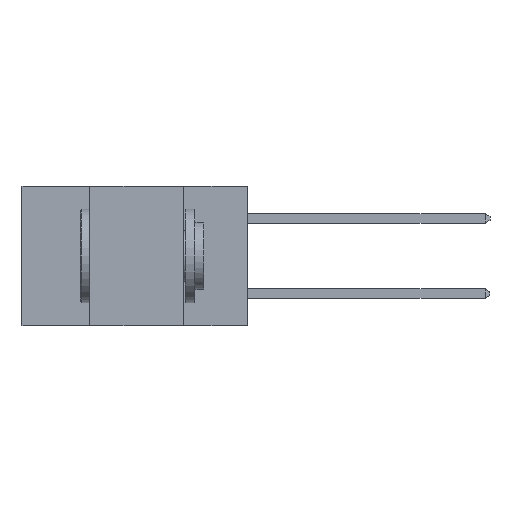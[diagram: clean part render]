
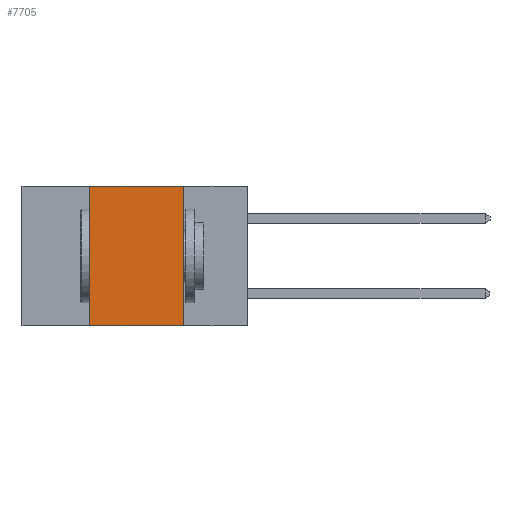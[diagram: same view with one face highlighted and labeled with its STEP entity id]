
A CAD part, left-side view. The second image highlights one B-rep face of the part: STEP entity #7705.
In plain terms, the highlighted planar face has unit normal (-1, 0, 0).
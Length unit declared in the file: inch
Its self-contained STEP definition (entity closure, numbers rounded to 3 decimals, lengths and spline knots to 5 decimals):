
#313 = CARTESIAN_POINT ( 'NONE',  ( 0., 0.42, 0. ) ) ;
#503 = LINE ( 'NONE', #12919, #856 ) ;
#856 = VECTOR ( 'NONE', #7271, 39.37008 ) ;
#1148 = CARTESIAN_POINT ( 'NONE',  ( 0., 0.6, 0. ) ) ;
#1267 = DIRECTION ( 'NONE',  ( 0., -1., 0. ) ) ;
#2216 = ORIENTED_EDGE ( 'NONE', *, *, #10490, .T. ) ;
#2292 = DIRECTION ( 'NONE',  ( 1., 0., 0. ) ) ;
#2371 = LINE ( 'NONE', #6980, #10793 ) ;
#2666 = ORIENTED_EDGE ( 'NONE', *, *, #11718, .F. ) ;
#3944 = ORIENTED_EDGE ( 'NONE', *, *, #7884, .F. ) ;
#4362 = FACE_OUTER_BOUND ( 'NONE', #4549, .T. ) ;
#4549 = EDGE_LOOP ( 'NONE', ( #2666, #12863, #3944, #2216 ) ) ;
#4908 = LINE ( 'NONE', #313, #13597 ) ;
#5125 = CARTESIAN_POINT ( 'NONE',  ( 0., 0.42, -0.37 ) ) ;
#6161 = DIRECTION ( 'NONE',  ( 0., -1., 0. ) ) ;
#6980 = CARTESIAN_POINT ( 'NONE',  ( 0., 0.6, 0. ) ) ;
#7162 = DIRECTION ( 'NONE',  ( 0., 0., 1. ) ) ;
#7271 = DIRECTION ( 'NONE',  ( 0., 0., -1. ) ) ;
#7454 = CARTESIAN_POINT ( 'NONE',  ( 0., 0.42, 0. ) ) ;
#7705 = ADVANCED_FACE ( 'NONE', ( #4362 ), #8005, .F. ) ;
#7884 = EDGE_CURVE ( 'NONE', #10605, #7950, #4908, .T. ) ;
#7950 = VERTEX_POINT ( 'NONE', #7454 ) ;
#8005 = PLANE ( 'NONE',  #14009 ) ;
#8231 = LINE ( 'NONE', #12992, #8577 ) ;
#8285 = CARTESIAN_POINT ( 'NONE',  ( 0., 0.17, -0.37 ) ) ;
#8386 = VERTEX_POINT ( 'NONE', #8285 ) ;
#8577 = VECTOR ( 'NONE', #6161, 39.37008 ) ;
#8952 = EDGE_CURVE ( 'NONE', #7950, #9631, #2371, .T. ) ;
#9631 = VERTEX_POINT ( 'NONE', #13715 ) ;
#10334 = DIRECTION ( 'NONE',  ( 0., 0., -1. ) ) ;
#10490 = EDGE_CURVE ( 'NONE', #10605, #8386, #8231, .T. ) ;
#10605 = VERTEX_POINT ( 'NONE', #5125 ) ;
#10793 = VECTOR ( 'NONE', #1267, 39.37008 ) ;
#11718 = EDGE_CURVE ( 'NONE', #9631, #8386, #503, .T. ) ;
#12863 = ORIENTED_EDGE ( 'NONE', *, *, #8952, .F. ) ;
#12919 = CARTESIAN_POINT ( 'NONE',  ( 0., 0.17, 0. ) ) ;
#12992 = CARTESIAN_POINT ( 'NONE',  ( 0., 0.6, -0.37 ) ) ;
#13597 = VECTOR ( 'NONE', #7162, 39.37008 ) ;
#13715 = CARTESIAN_POINT ( 'NONE',  ( 0., 0.17, 0. ) ) ;
#14009 = AXIS2_PLACEMENT_3D ( 'NONE', #1148, #2292, #10334 ) ;
